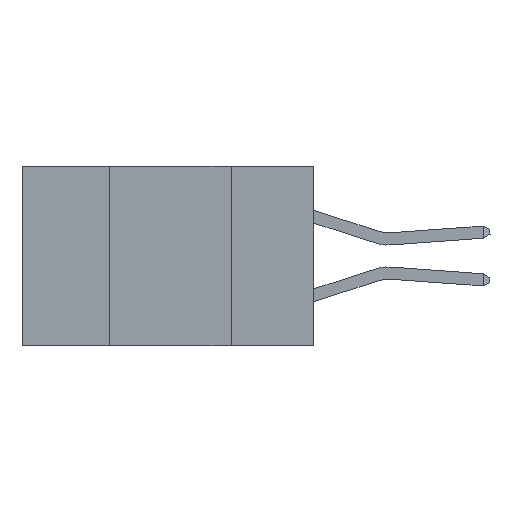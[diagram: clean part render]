
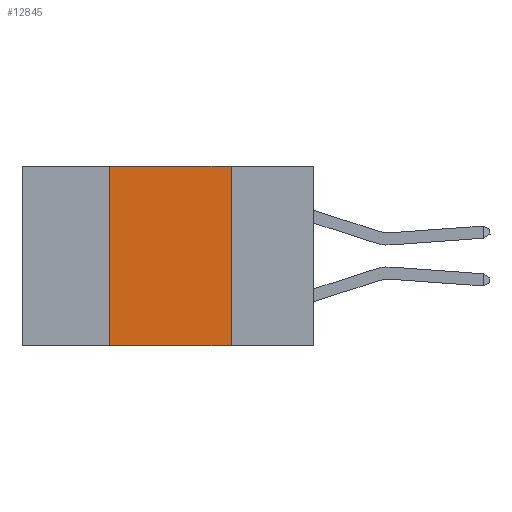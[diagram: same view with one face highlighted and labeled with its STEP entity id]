
A CAD part, left-side view. The second image highlights one B-rep face of the part: STEP entity #12845.
In plain terms, the highlighted planar face has unit normal (-1, 0, 0).
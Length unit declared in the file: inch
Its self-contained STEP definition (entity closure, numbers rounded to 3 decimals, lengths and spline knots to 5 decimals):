
#1032 = VECTOR ( 'NONE', #12225, 39.37008 ) ;
#1114 = EDGE_CURVE ( 'NONE', #12140, #2739, #3839, .T. ) ;
#1147 = EDGE_CURVE ( 'NONE', #4423, #4073, #1670, .T. ) ;
#1670 = LINE ( 'NONE', #5038, #14057 ) ;
#1693 = EDGE_LOOP ( 'NONE', ( #5298, #5016, #10244, #8151 ) ) ;
#1786 = AXIS2_PLACEMENT_3D ( 'NONE', #6182, #5279, #3043 ) ;
#2224 = CARTESIAN_POINT ( 'NONE',  ( 0., 0.42, -0.37 ) ) ;
#2275 = CARTESIAN_POINT ( 'NONE',  ( 0., 0.17, 0. ) ) ;
#2739 = VERTEX_POINT ( 'NONE', #10791 ) ;
#3043 = DIRECTION ( 'NONE',  ( 0., 0., -1. ) ) ;
#3566 = FACE_OUTER_BOUND ( 'NONE', #1693, .T. ) ;
#3839 = LINE ( 'NONE', #8394, #12649 ) ;
#4073 = VERTEX_POINT ( 'NONE', #13096 ) ;
#4423 = VERTEX_POINT ( 'NONE', #2275 ) ;
#5016 = ORIENTED_EDGE ( 'NONE', *, *, #11114, .F. ) ;
#5038 = CARTESIAN_POINT ( 'NONE',  ( 0., 0.17, 0. ) ) ;
#5279 = DIRECTION ( 'NONE',  ( 1., 0., 0. ) ) ;
#5298 = ORIENTED_EDGE ( 'NONE', *, *, #1147, .F. ) ;
#5892 = PLANE ( 'NONE',  #1786 ) ;
#6182 = CARTESIAN_POINT ( 'NONE',  ( 0., 0.6, 0. ) ) ;
#6483 = LINE ( 'NONE', #12336, #10583 ) ;
#7636 = CARTESIAN_POINT ( 'NONE',  ( 0., 0.6, 0. ) ) ;
#7815 = DIRECTION ( 'NONE',  ( 0., -1., 0. ) ) ;
#8151 = ORIENTED_EDGE ( 'NONE', *, *, #10820, .T. ) ;
#8394 = CARTESIAN_POINT ( 'NONE',  ( 0., 0.42, 0. ) ) ;
#9472 = LINE ( 'NONE', #7636, #1032 ) ;
#10244 = ORIENTED_EDGE ( 'NONE', *, *, #1114, .F. ) ;
#10583 = VECTOR ( 'NONE', #7815, 39.37008 ) ;
#10655 = DIRECTION ( 'NONE',  ( 0., 0., -1. ) ) ;
#10791 = CARTESIAN_POINT ( 'NONE',  ( 0., 0.42, 0. ) ) ;
#10820 = EDGE_CURVE ( 'NONE', #12140, #4073, #6483, .T. ) ;
#11114 = EDGE_CURVE ( 'NONE', #2739, #4423, #9472, .T. ) ;
#12140 = VERTEX_POINT ( 'NONE', #2224 ) ;
#12225 = DIRECTION ( 'NONE',  ( 0., -1., 0. ) ) ;
#12336 = CARTESIAN_POINT ( 'NONE',  ( 0., 0.6, -0.37 ) ) ;
#12649 = VECTOR ( 'NONE', #14015, 39.37008 ) ;
#12845 = ADVANCED_FACE ( 'NONE', ( #3566 ), #5892, .F. ) ;
#13096 = CARTESIAN_POINT ( 'NONE',  ( 0., 0.17, -0.37 ) ) ;
#14015 = DIRECTION ( 'NONE',  ( 0., 0., 1. ) ) ;
#14057 = VECTOR ( 'NONE', #10655, 39.37008 ) ;
